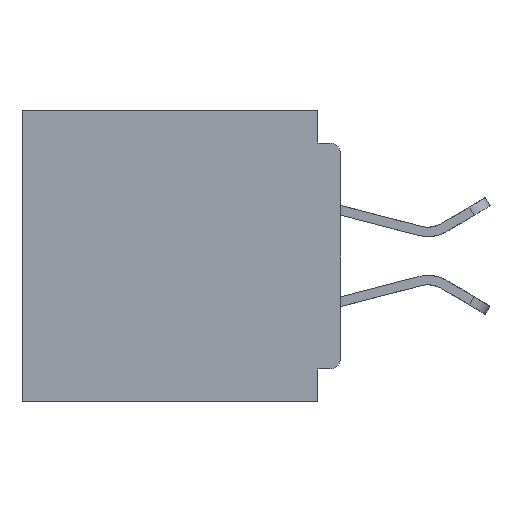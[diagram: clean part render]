
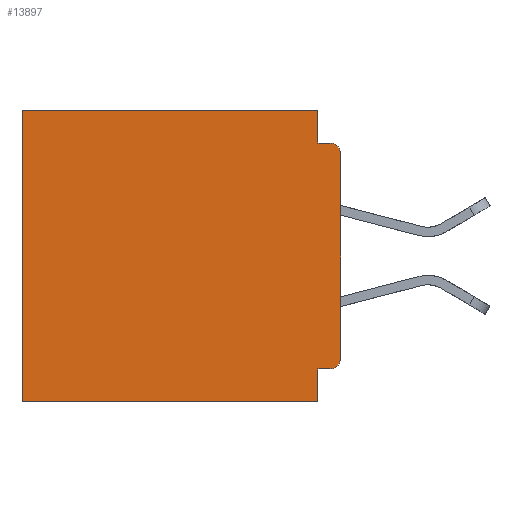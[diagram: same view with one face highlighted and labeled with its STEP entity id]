
A CAD part, left-side view. The second image highlights one B-rep face of the part: STEP entity #13897.
In plain terms, the highlighted planar face has unit normal (-1, 0, 0).
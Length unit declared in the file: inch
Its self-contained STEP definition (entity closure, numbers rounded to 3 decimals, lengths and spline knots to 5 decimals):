
#264 = ORIENTED_EDGE ( 'NONE', *, *, #4230, .T. ) ;
#648 = CARTESIAN_POINT ( 'NONE',  ( 0.3, 0., 0. ) ) ;
#1986 = LINE ( 'NONE', #3784, #30714 ) ;
#1991 = CARTESIAN_POINT ( 'NONE',  ( 0.3, 0., -0.4 ) ) ;
#2714 = ORIENTED_EDGE ( 'NONE', *, *, #8604, .F. ) ;
#3345 = VERTEX_POINT ( 'NONE', #10842 ) ;
#3784 = CARTESIAN_POINT ( 'NONE',  ( 0.3, 0., -0.355 ) ) ;
#3873 = VECTOR ( 'NONE', #33001, 39.37008 ) ;
#3941 = CIRCLE ( 'NONE', #13809, 0.015 ) ;
#3955 = CARTESIAN_POINT ( 'NONE',  ( 0.3, 0.031, -0.4 ) ) ;
#4210 = DIRECTION ( 'NONE',  ( 0., 0., -1. ) ) ;
#4230 = EDGE_CURVE ( 'NONE', #33134, #28975, #28989, .T. ) ;
#4298 = VECTOR ( 'NONE', #6805, 39.37008 ) ;
#4829 = LINE ( 'NONE', #32235, #33381 ) ;
#5156 = LINE ( 'NONE', #3955, #4298 ) ;
#5336 = ORIENTED_EDGE ( 'NONE', *, *, #14456, .T. ) ;
#6473 = CARTESIAN_POINT ( 'NONE',  ( 0.3, 0.031, -0.4 ) ) ;
#6805 = DIRECTION ( 'NONE',  ( 0., 0., -1. ) ) ;
#7188 = VECTOR ( 'NONE', #15098, 39.37008 ) ;
#7319 = DIRECTION ( 'NONE',  ( -1., 0., 0. ) ) ;
#7599 = CARTESIAN_POINT ( 'NONE',  ( 0.3, 0.015, -0.045 ) ) ;
#7932 = AXIS2_PLACEMENT_3D ( 'NONE', #10480, #29706, #13289 ) ;
#8604 = EDGE_CURVE ( 'NONE', #19433, #18199, #4829, .T. ) ;
#8986 = VERTEX_POINT ( 'NONE', #23375 ) ;
#10480 = CARTESIAN_POINT ( 'NONE',  ( 0.3, 0.015, -0.06 ) ) ;
#10602 = PLANE ( 'NONE',  #17100 ) ;
#10842 = CARTESIAN_POINT ( 'NONE',  ( 0.3, 0., -0.06 ) ) ;
#13289 = DIRECTION ( 'NONE',  ( 0., 0., -1. ) ) ;
#13434 = DIRECTION ( 'NONE',  ( 1., 0., 0. ) ) ;
#13809 = AXIS2_PLACEMENT_3D ( 'NONE', #23942, #7319, #26697 ) ;
#13897 = ADVANCED_FACE ( 'NONE', ( #27886 ), #10602, .F. ) ;
#13909 = CARTESIAN_POINT ( 'NONE',  ( 0.3, 0., -0.4 ) ) ;
#13917 = EDGE_CURVE ( 'NONE', #33034, #28975, #21482, .T. ) ;
#14456 = EDGE_CURVE ( 'NONE', #22982, #16624, #3941, .T. ) ;
#14619 = ORIENTED_EDGE ( 'NONE', *, *, #24733, .F. ) ;
#15098 = DIRECTION ( 'NONE',  ( 0., -1., 0. ) ) ;
#16544 = ORIENTED_EDGE ( 'NONE', *, *, #17590, .T. ) ;
#16624 = VERTEX_POINT ( 'NONE', #23959 ) ;
#17100 = AXIS2_PLACEMENT_3D ( 'NONE', #1991, #13434, #32566 ) ;
#17590 = EDGE_CURVE ( 'NONE', #3345, #30431, #34593, .T. ) ;
#18061 = EDGE_CURVE ( 'NONE', #8986, #33034, #5156, .T. ) ;
#18199 = VERTEX_POINT ( 'NONE', #24961 ) ;
#19433 = VERTEX_POINT ( 'NONE', #33768 ) ;
#20771 = CARTESIAN_POINT ( 'NONE',  ( 0.3, 0.437, -0.4 ) ) ;
#20800 = EDGE_CURVE ( 'NONE', #18199, #30431, #22014, .T. ) ;
#21482 = LINE ( 'NONE', #35264, #34250 ) ;
#21730 = DIRECTION ( 'NONE',  ( 0., 1., 0. ) ) ;
#21881 = CARTESIAN_POINT ( 'NONE',  ( 0.3, 0.015, -0.355 ) ) ;
#22014 = LINE ( 'NONE', #34155, #7188 ) ;
#22982 = VERTEX_POINT ( 'NONE', #21881 ) ;
#23101 = DIRECTION ( 'NONE',  ( 0., 1., 0. ) ) ;
#23349 = ORIENTED_EDGE ( 'NONE', *, *, #20800, .F. ) ;
#23375 = CARTESIAN_POINT ( 'NONE',  ( 0.3, 0.031, -0.355 ) ) ;
#23847 = ORIENTED_EDGE ( 'NONE', *, *, #13917, .F. ) ;
#23942 = CARTESIAN_POINT ( 'NONE',  ( 0.3, 0.015, -0.34 ) ) ;
#23959 = CARTESIAN_POINT ( 'NONE',  ( 0.3, 0., -0.34 ) ) ;
#24733 = EDGE_CURVE ( 'NONE', #3345, #16624, #31614, .T. ) ;
#24790 = VECTOR ( 'NONE', #23101, 39.37008 ) ;
#24961 = CARTESIAN_POINT ( 'NONE',  ( 0.3, 0.031, -0.045 ) ) ;
#24980 = EDGE_CURVE ( 'NONE', #19433, #33134, #31177, .T. ) ;
#25637 = EDGE_CURVE ( 'NONE', #22982, #8986, #1986, .T. ) ;
#26697 = DIRECTION ( 'NONE',  ( 0., 0., -1. ) ) ;
#27886 = FACE_OUTER_BOUND ( 'NONE', #28529, .T. ) ;
#28529 = EDGE_LOOP ( 'NONE', ( #14619, #16544, #23349, #2714, #31520, #264, #23847, #29789, #30612, #5336 ) ) ;
#28782 = DIRECTION ( 'NONE',  ( 0., 1., 0. ) ) ;
#28975 = VERTEX_POINT ( 'NONE', #20771 ) ;
#28989 = LINE ( 'NONE', #29427, #29853 ) ;
#29427 = CARTESIAN_POINT ( 'NONE',  ( 0.3, 0.437, -0.4 ) ) ;
#29706 = DIRECTION ( 'NONE',  ( -1., 0., 0. ) ) ;
#29789 = ORIENTED_EDGE ( 'NONE', *, *, #18061, .F. ) ;
#29853 = VECTOR ( 'NONE', #4210, 39.37008 ) ;
#30431 = VERTEX_POINT ( 'NONE', #7599 ) ;
#30612 = ORIENTED_EDGE ( 'NONE', *, *, #25637, .F. ) ;
#30714 = VECTOR ( 'NONE', #28782, 39.37008 ) ;
#31177 = LINE ( 'NONE', #648, #24790 ) ;
#31520 = ORIENTED_EDGE ( 'NONE', *, *, #24980, .T. ) ;
#31614 = LINE ( 'NONE', #13909, #3873 ) ;
#32235 = CARTESIAN_POINT ( 'NONE',  ( 0.3, 0.031, 0. ) ) ;
#32566 = DIRECTION ( 'NONE',  ( 0., 0., -1. ) ) ;
#33001 = DIRECTION ( 'NONE',  ( 0., 0., -1. ) ) ;
#33034 = VERTEX_POINT ( 'NONE', #6473 ) ;
#33134 = VERTEX_POINT ( 'NONE', #34443 ) ;
#33381 = VECTOR ( 'NONE', #33420, 39.37008 ) ;
#33420 = DIRECTION ( 'NONE',  ( 0., 0., -1. ) ) ;
#33768 = CARTESIAN_POINT ( 'NONE',  ( 0.3, 0.031, 0. ) ) ;
#34155 = CARTESIAN_POINT ( 'NONE',  ( 0.3, 0., -0.045 ) ) ;
#34250 = VECTOR ( 'NONE', #21730, 39.37008 ) ;
#34443 = CARTESIAN_POINT ( 'NONE',  ( 0.3, 0.437, 0. ) ) ;
#34593 = CIRCLE ( 'NONE', #7932, 0.015 ) ;
#35264 = CARTESIAN_POINT ( 'NONE',  ( 0.3, 0., -0.4 ) ) ;
